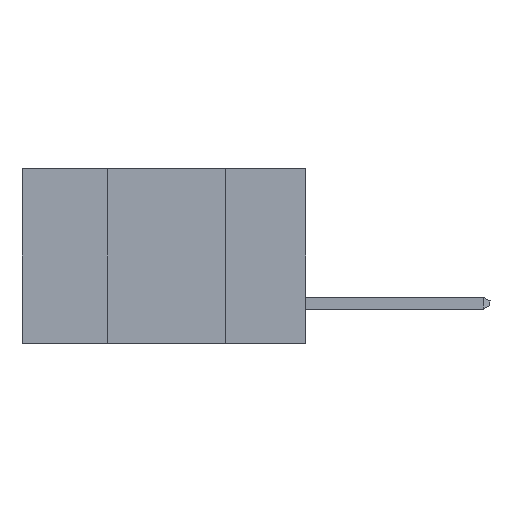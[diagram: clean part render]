
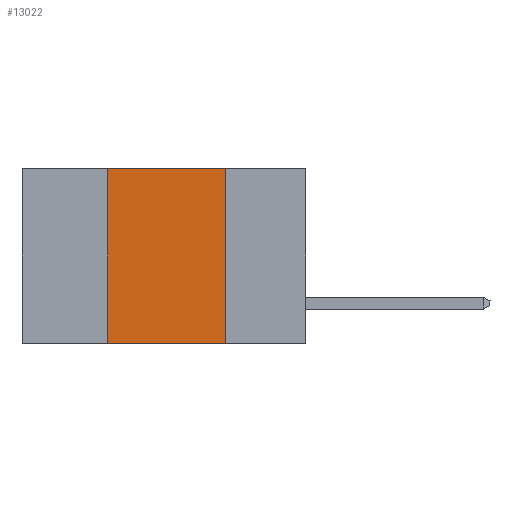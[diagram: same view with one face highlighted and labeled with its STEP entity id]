
A CAD part, left-side view. The second image highlights one B-rep face of the part: STEP entity #13022.
In plain terms, the highlighted planar face has unit normal (-1, 0, 0).
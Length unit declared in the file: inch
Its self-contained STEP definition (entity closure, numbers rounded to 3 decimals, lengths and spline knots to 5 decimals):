
#1501 = VECTOR ( 'NONE', #10834, 39.37008 ) ;
#2273 = CARTESIAN_POINT ( 'NONE',  ( 0., 0.17, 0. ) ) ;
#2426 = LINE ( 'NONE', #3586, #1501 ) ;
#2786 = LINE ( 'NONE', #13256, #10695 ) ;
#2863 = VERTEX_POINT ( 'NONE', #4863 ) ;
#2939 = ORIENTED_EDGE ( 'NONE', *, *, #8680, .F. ) ;
#3319 = VERTEX_POINT ( 'NONE', #10311 ) ;
#3546 = DIRECTION ( 'NONE',  ( 1., 0., 0. ) ) ;
#3586 = CARTESIAN_POINT ( 'NONE',  ( 0., 0.17, -0.37 ) ) ;
#3610 = CARTESIAN_POINT ( 'NONE',  ( 0., 0.6, 0. ) ) ;
#3905 = EDGE_CURVE ( 'NONE', #11231, #8633, #2426, .T. ) ;
#4294 = CARTESIAN_POINT ( 'NONE',  ( 0., 0.6, 0. ) ) ;
#4597 = EDGE_CURVE ( 'NONE', #3319, #2863, #2786, .T. ) ;
#4863 = CARTESIAN_POINT ( 'NONE',  ( 0., 0.42, 0. ) ) ;
#5949 = AXIS2_PLACEMENT_3D ( 'NONE', #3610, #3546, #12929 ) ;
#6411 = DIRECTION ( 'NONE',  ( 0., -1., 0. ) ) ;
#7037 = DIRECTION ( 'NONE',  ( 0., 0., 1. ) ) ;
#7260 = ORIENTED_EDGE ( 'NONE', *, *, #4597, .F. ) ;
#7478 = VECTOR ( 'NONE', #6411, 39.37008 ) ;
#7510 = CARTESIAN_POINT ( 'NONE',  ( 0., 0.6, -0.37 ) ) ;
#8297 = VECTOR ( 'NONE', #8469, 39.37008 ) ;
#8469 = DIRECTION ( 'NONE',  ( 0., -1., 0. ) ) ;
#8633 = VERTEX_POINT ( 'NONE', #12111 ) ;
#8680 = EDGE_CURVE ( 'NONE', #2863, #11231, #13537, .T. ) ;
#8814 = PLANE ( 'NONE',  #5949 ) ;
#8875 = FACE_OUTER_BOUND ( 'NONE', #9010, .T. ) ;
#9010 = EDGE_LOOP ( 'NONE', ( #11079, #2939, #7260, #10024 ) ) ;
#10024 = ORIENTED_EDGE ( 'NONE', *, *, #12012, .T. ) ;
#10311 = CARTESIAN_POINT ( 'NONE',  ( 0., 0.42, -0.37 ) ) ;
#10695 = VECTOR ( 'NONE', #7037, 39.37008 ) ;
#10834 = DIRECTION ( 'NONE',  ( 0., 0., -1. ) ) ;
#11079 = ORIENTED_EDGE ( 'NONE', *, *, #3905, .F. ) ;
#11231 = VERTEX_POINT ( 'NONE', #2273 ) ;
#11539 = LINE ( 'NONE', #7510, #7478 ) ;
#12012 = EDGE_CURVE ( 'NONE', #3319, #8633, #11539, .T. ) ;
#12111 = CARTESIAN_POINT ( 'NONE',  ( 0., 0.17, -0.37 ) ) ;
#12929 = DIRECTION ( 'NONE',  ( 0., 0., -1. ) ) ;
#13022 = ADVANCED_FACE ( 'NONE', ( #8875 ), #8814, .F. ) ;
#13256 = CARTESIAN_POINT ( 'NONE',  ( 0., 0.42, -0.37 ) ) ;
#13537 = LINE ( 'NONE', #4294, #8297 ) ;
